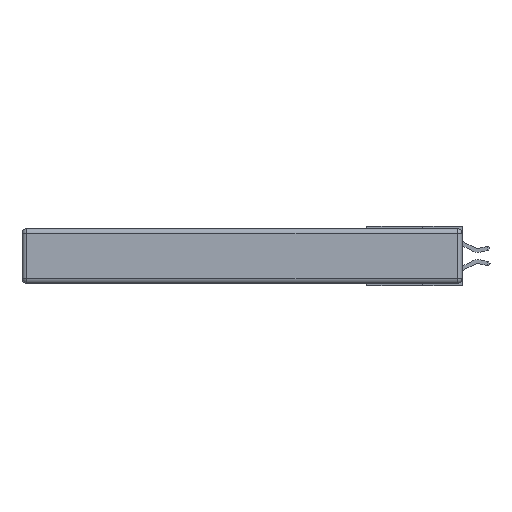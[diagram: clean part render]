
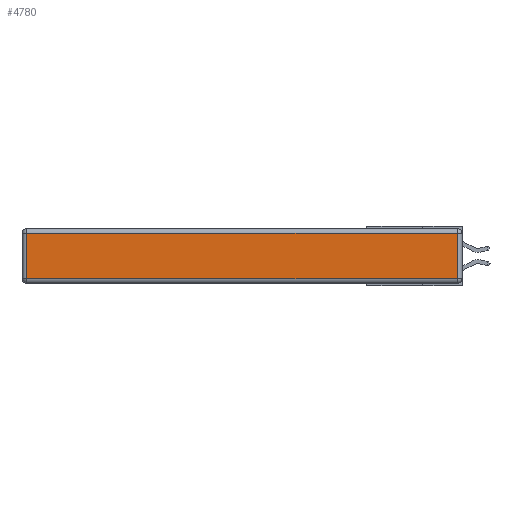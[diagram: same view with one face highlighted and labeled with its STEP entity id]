
A CAD part, left-side view. The second image highlights one B-rep face of the part: STEP entity #4780.
In plain terms, the highlighted planar face has unit normal (-1, 0, 0).
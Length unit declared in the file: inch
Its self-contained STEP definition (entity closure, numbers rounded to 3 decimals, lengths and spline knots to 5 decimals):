
#18 = CARTESIAN_POINT ( 'NONE',  ( 0., 0., -0.313 ) ) ;
#386 = VECTOR ( 'NONE', #14612, 39.37008 ) ;
#503 = VECTOR ( 'NONE', #7366, 39.37008 ) ;
#513 = EDGE_CURVE ( 'NONE', #5132, #5228, #10783, .T. ) ;
#570 = EDGE_CURVE ( 'NONE', #5228, #2087, #4166, .T. ) ;
#656 = CARTESIAN_POINT ( 'NONE',  ( 0., 2.72, -0.03 ) ) ;
#867 = VERTEX_POINT ( 'NONE', #1728 ) ;
#1728 = CARTESIAN_POINT ( 'NONE',  ( 0., 2.72, -0.313 ) ) ;
#2087 = VERTEX_POINT ( 'NONE', #656 ) ;
#3205 = LINE ( 'NONE', #3977, #503 ) ;
#3977 = CARTESIAN_POINT ( 'NONE',  ( 0., 2.72, -0.343 ) ) ;
#4166 = LINE ( 'NONE', #6565, #386 ) ;
#4170 = CARTESIAN_POINT ( 'NONE',  ( 0., 0.03, -0.343 ) ) ;
#4325 = EDGE_CURVE ( 'NONE', #867, #5132, #14413, .T. ) ;
#4352 = EDGE_LOOP ( 'NONE', ( #4865, #14322, #8993, #12876 ) ) ;
#4780 = ADVANCED_FACE ( 'NONE', ( #12624 ), #5294, .T. ) ;
#4865 = ORIENTED_EDGE ( 'NONE', *, *, #4325, .T. ) ;
#5132 = VERTEX_POINT ( 'NONE', #6139 ) ;
#5228 = VERTEX_POINT ( 'NONE', #14327 ) ;
#5294 = PLANE ( 'NONE',  #11964 ) ;
#5751 = DIRECTION ( 'NONE',  ( 0., -1., 0. ) ) ;
#6139 = CARTESIAN_POINT ( 'NONE',  ( 0., 0.03, -0.313 ) ) ;
#6565 = CARTESIAN_POINT ( 'NONE',  ( 0., 2.75, -0.03 ) ) ;
#7125 = EDGE_CURVE ( 'NONE', #2087, #867, #3205, .T. ) ;
#7366 = DIRECTION ( 'NONE',  ( 0., 0., -1. ) ) ;
#7560 = VECTOR ( 'NONE', #5751, 39.37008 ) ;
#7671 = CARTESIAN_POINT ( 'NONE',  ( 0., 0., -0.343 ) ) ;
#7750 = VECTOR ( 'NONE', #12181, 39.37008 ) ;
#8993 = ORIENTED_EDGE ( 'NONE', *, *, #570, .T. ) ;
#9926 = DIRECTION ( 'NONE',  ( 0., 0., 1. ) ) ;
#10783 = LINE ( 'NONE', #4170, #7750 ) ;
#11964 = AXIS2_PLACEMENT_3D ( 'NONE', #7671, #13461, #9926 ) ;
#12181 = DIRECTION ( 'NONE',  ( 0., 0., 1. ) ) ;
#12624 = FACE_OUTER_BOUND ( 'NONE', #4352, .T. ) ;
#12876 = ORIENTED_EDGE ( 'NONE', *, *, #7125, .T. ) ;
#13461 = DIRECTION ( 'NONE',  ( -1., 0., 0. ) ) ;
#14322 = ORIENTED_EDGE ( 'NONE', *, *, #513, .T. ) ;
#14327 = CARTESIAN_POINT ( 'NONE',  ( 0., 0.03, -0.03 ) ) ;
#14413 = LINE ( 'NONE', #18, #7560 ) ;
#14612 = DIRECTION ( 'NONE',  ( 0., 1., 0. ) ) ;
